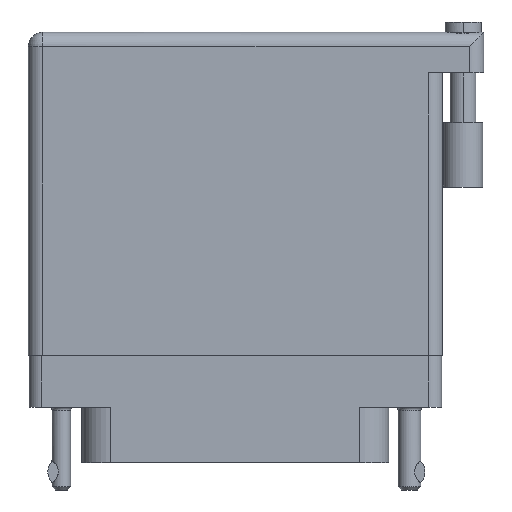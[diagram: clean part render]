
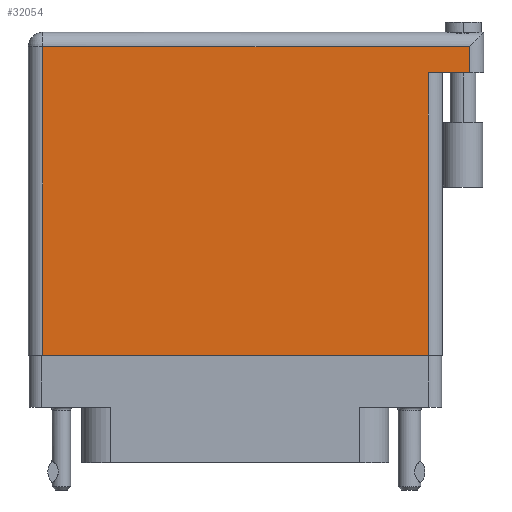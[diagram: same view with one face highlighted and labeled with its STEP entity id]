
A CAD part, front view. The second image highlights one B-rep face of the part: STEP entity #32054.
In plain terms, the highlighted face is planar.
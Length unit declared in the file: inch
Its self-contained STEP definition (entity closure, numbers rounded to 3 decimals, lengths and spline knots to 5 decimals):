
#940 = VECTOR ( 'NONE', #37558, 39.37008 ) ;
#2906 = ORIENTED_EDGE ( 'NONE', *, *, #46310, .F. ) ;
#2926 = VECTOR ( 'NONE', #29727, 39.37008 ) ;
#4377 = CARTESIAN_POINT ( 'NONE',  ( 0.934, 1.269, 0.4495 ) ) ;
#6322 = DIRECTION ( 'NONE',  ( 0., 0., -1. ) ) ;
#6957 = CARTESIAN_POINT ( 'NONE',  ( 0.934, -0.1, 0.4495 ) ) ;
#7350 = VECTOR ( 'NONE', #42128, 39.37008 ) ;
#7600 = VECTOR ( 'NONE', #46740, 39.37008 ) ;
#9267 = CARTESIAN_POINT ( 'NONE',  ( 0.934, 1.269, 0.4495 ) ) ;
#9774 = LINE ( 'NONE', #44741, #16813 ) ;
#9930 = CARTESIAN_POINT ( 'NONE',  ( -0.934, 1.396, 0.4495 ) ) ;
#10222 = EDGE_CURVE ( 'NONE', #23348, #48498, #9774, .T. ) ;
#12066 = CARTESIAN_POINT ( 'NONE',  ( 1.134, 1.466, 0.4495 ) ) ;
#13294 = LINE ( 'NONE', #22342, #940 ) ;
#15584 = LINE ( 'NONE', #12066, #38682 ) ;
#16251 = EDGE_CURVE ( 'NONE', #48498, #18533, #34757, .T. ) ;
#16813 = VECTOR ( 'NONE', #22607, 39.37008 ) ;
#17362 = LINE ( 'NONE', #34663, #7350 ) ;
#18457 = ORIENTED_EDGE ( 'NONE', *, *, #18863, .T. ) ;
#18533 = VERTEX_POINT ( 'NONE', #9267 ) ;
#18651 = VERTEX_POINT ( 'NONE', #9930 ) ;
#18863 = EDGE_CURVE ( 'NONE', #32667, #48142, #15584, .T. ) ;
#19403 = ORIENTED_EDGE ( 'NONE', *, *, #10222, .T. ) ;
#22342 = CARTESIAN_POINT ( 'NONE',  ( 1.204, 1.269, 0.4495 ) ) ;
#22513 = CARTESIAN_POINT ( 'NONE',  ( 1.134, 1.396, 0.4495 ) ) ;
#22607 = DIRECTION ( 'NONE',  ( 1., 0., 0. ) ) ;
#23348 = VERTEX_POINT ( 'NONE', #38286 ) ;
#25455 = EDGE_CURVE ( 'NONE', #18651, #23348, #46596, .T. ) ;
#27210 = ORIENTED_EDGE ( 'NONE', *, *, #31330, .T. ) ;
#28896 = CARTESIAN_POINT ( 'NONE',  ( -1.004, 1.466, 0.4495 ) ) ;
#29380 = CARTESIAN_POINT ( 'NONE',  ( -0.934, -0.1, 0.4495 ) ) ;
#29727 = DIRECTION ( 'NONE',  ( 0., -1., 0. ) ) ;
#31330 = EDGE_CURVE ( 'NONE', #48142, #18651, #17362, .T. ) ;
#32054 = ADVANCED_FACE ( 'NONE', ( #34421 ), #47765, .F. ) ;
#32228 = DIRECTION ( 'NONE',  ( -1., 0., 0. ) ) ;
#32667 = VERTEX_POINT ( 'NONE', #41076 ) ;
#33111 = AXIS2_PLACEMENT_3D ( 'NONE', #28896, #6322, #32228 ) ;
#34421 = FACE_OUTER_BOUND ( 'NONE', #43141, .T. ) ;
#34663 = CARTESIAN_POINT ( 'NONE',  ( -1.004, 1.396, 0.4495 ) ) ;
#34757 = LINE ( 'NONE', #4377, #7600 ) ;
#34825 = DIRECTION ( 'NONE',  ( 0., 1., 0. ) ) ;
#37558 = DIRECTION ( 'NONE',  ( -1., 0., 0. ) ) ;
#38286 = CARTESIAN_POINT ( 'NONE',  ( -0.934, -0.1, 0.4495 ) ) ;
#38682 = VECTOR ( 'NONE', #34825, 39.37008 ) ;
#39398 = ORIENTED_EDGE ( 'NONE', *, *, #25455, .T. ) ;
#41076 = CARTESIAN_POINT ( 'NONE',  ( 1.134, 1.269, 0.4495 ) ) ;
#42128 = DIRECTION ( 'NONE',  ( -1., 0., 0. ) ) ;
#43141 = EDGE_LOOP ( 'NONE', ( #19403, #48322, #2906, #18457, #27210, #39398 ) ) ;
#44741 = CARTESIAN_POINT ( 'NONE',  ( -1.004, -0.1, 0.4495 ) ) ;
#46310 = EDGE_CURVE ( 'NONE', #32667, #18533, #13294, .T. ) ;
#46596 = LINE ( 'NONE', #29380, #2926 ) ;
#46740 = DIRECTION ( 'NONE',  ( 0., 1., 0. ) ) ;
#47765 = PLANE ( 'NONE',  #33111 ) ;
#48142 = VERTEX_POINT ( 'NONE', #22513 ) ;
#48322 = ORIENTED_EDGE ( 'NONE', *, *, #16251, .T. ) ;
#48498 = VERTEX_POINT ( 'NONE', #6957 ) ;
